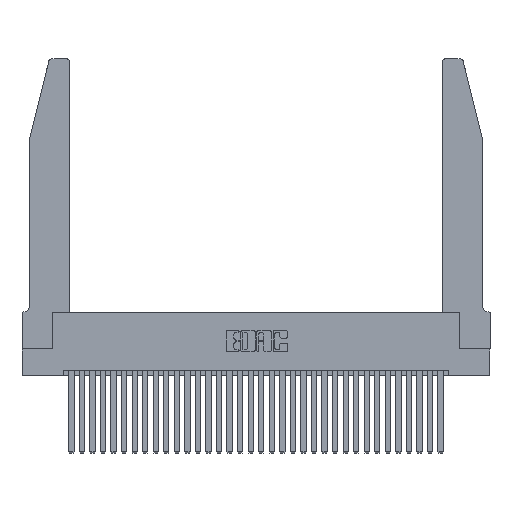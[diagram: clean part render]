
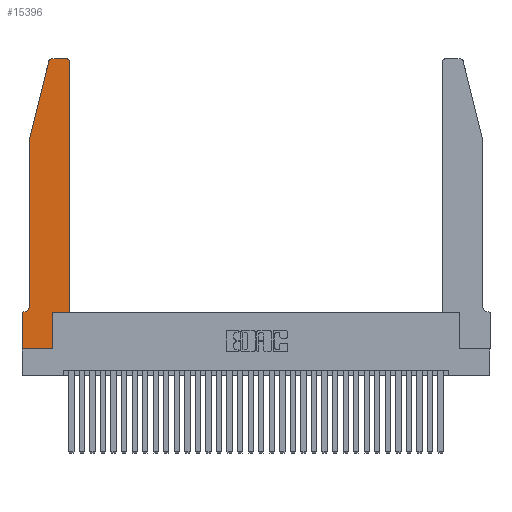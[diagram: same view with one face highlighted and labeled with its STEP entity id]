
A CAD part, top view. The second image highlights one B-rep face of the part: STEP entity #15396.
In plain terms, the highlighted planar face has unit normal (0, 0, 1).
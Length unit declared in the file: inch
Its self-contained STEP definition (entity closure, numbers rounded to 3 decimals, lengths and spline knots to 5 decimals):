
#211 = DIRECTION ( 'NONE',  ( 1., 0., 0. ) ) ;
#323 = DIRECTION ( 'NONE',  ( 1., 0., 0. ) ) ;
#579 = EDGE_CURVE ( 'NONE', #9746, #6793, #3070, .T. ) ;
#960 = ORIENTED_EDGE ( 'NONE', *, *, #579, .T. ) ;
#1198 = LINE ( 'NONE', #16739, #21111 ) ;
#2134 = DIRECTION ( 'NONE',  ( 0., 0., -1. ) ) ;
#2361 = EDGE_CURVE ( 'NONE', #6656, #9746, #30515, .T. ) ;
#2761 = EDGE_CURVE ( 'NONE', #21842, #29448, #1198, .T. ) ;
#3023 = CIRCLE ( 'NONE', #4635, 0.03 ) ;
#3070 = LINE ( 'NONE', #5357, #6378 ) ;
#3404 = CARTESIAN_POINT ( 'NONE',  ( 0., 0., 0.37 ) ) ;
#3480 = LINE ( 'NONE', #3404, #15290 ) ;
#3879 = DIRECTION ( 'NONE',  ( -1., 0., 0. ) ) ;
#4460 = DIRECTION ( 'NONE',  ( 0., 1., 0. ) ) ;
#4463 = CARTESIAN_POINT ( 'NONE',  ( 0., 0.35, 0.37 ) ) ;
#4635 = AXIS2_PLACEMENT_3D ( 'NONE', #15820, #31505, #323 ) ;
#4909 = DIRECTION ( 'NONE',  ( 1., 0., 0. ) ) ;
#5357 = CARTESIAN_POINT ( 'NONE',  ( 0.4505, 0.35, 0.37 ) ) ;
#6378 = VECTOR ( 'NONE', #23825, 39.37008 ) ;
#6656 = VERTEX_POINT ( 'NONE', #24664 ) ;
#6670 = CARTESIAN_POINT ( 'NONE',  ( 0.25487, 2.72718, 0.37 ) ) ;
#6793 = VERTEX_POINT ( 'NONE', #17738 ) ;
#7742 = CARTESIAN_POINT ( 'NONE',  ( 0.0055, 0.35, 0.37 ) ) ;
#8192 = DIRECTION ( 'NONE',  ( 0., 0., 1. ) ) ;
#8232 = ORIENTED_EDGE ( 'NONE', *, *, #32897, .T. ) ;
#9725 = CIRCLE ( 'NONE', #13963, 0.03 ) ;
#9746 = VERTEX_POINT ( 'NONE', #15189 ) ;
#9823 = VECTOR ( 'NONE', #10952, 39.37008 ) ;
#10944 = EDGE_CURVE ( 'NONE', #14311, #14879, #15466, .T. ) ;
#10952 = DIRECTION ( 'NONE',  ( -0.239, -0.971, 0. ) ) ;
#12093 = CARTESIAN_POINT ( 'NONE',  ( 0.4505, 0.35, 0.37 ) ) ;
#12300 = DIRECTION ( 'NONE',  ( 0., 0., 1. ) ) ;
#12455 = FACE_OUTER_BOUND ( 'NONE', #14557, .T. ) ;
#12748 = VERTEX_POINT ( 'NONE', #31370 ) ;
#13379 = ORIENTED_EDGE ( 'NONE', *, *, #23040, .T. ) ;
#13963 = AXIS2_PLACEMENT_3D ( 'NONE', #25676, #12300, #4909 ) ;
#14055 = CARTESIAN_POINT ( 'NONE',  ( 0.284, 2.75, 0.37 ) ) ;
#14167 = ORIENTED_EDGE ( 'NONE', *, *, #19040, .T. ) ;
#14311 = VERTEX_POINT ( 'NONE', #19934 ) ;
#14557 = EDGE_LOOP ( 'NONE', ( #19829, #8232, #14167, #31690, #17922, #22378, #33277, #13379, #32469, #960, #21387, #23759 ) ) ;
#14879 = VERTEX_POINT ( 'NONE', #31973 ) ;
#15189 = CARTESIAN_POINT ( 'NONE',  ( 0.2865, 0.35, 0.37 ) ) ;
#15290 = VECTOR ( 'NONE', #21895, 39.37008 ) ;
#15393 = VECTOR ( 'NONE', #4460, 39.37008 ) ;
#15396 = ADVANCED_FACE ( 'NONE', ( #12455 ), #27158, .T. ) ;
#15466 = LINE ( 'NONE', #17640, #18686 ) ;
#15694 = CARTESIAN_POINT ( 'NONE',  ( 0.2865, 0.35, 0.37 ) ) ;
#15798 = CARTESIAN_POINT ( 'NONE',  ( 0., 0., 0.37 ) ) ;
#15820 = CARTESIAN_POINT ( 'NONE',  ( 0.4205, 2.72, 0.37 ) ) ;
#15999 = DIRECTION ( 'NONE',  ( 1., 0., 0. ) ) ;
#16010 = LINE ( 'NONE', #15798, #17278 ) ;
#16063 = VERTEX_POINT ( 'NONE', #28778 ) ;
#16739 = CARTESIAN_POINT ( 'NONE',  ( 0.0755, 0.35, 0.37 ) ) ;
#17278 = VECTOR ( 'NONE', #211, 39.37008 ) ;
#17640 = CARTESIAN_POINT ( 'NONE',  ( 0.0755, 2., 0.37 ) ) ;
#17738 = CARTESIAN_POINT ( 'NONE',  ( 0.4505, 0.35, 0.37 ) ) ;
#17922 = ORIENTED_EDGE ( 'NONE', *, *, #31210, .T. ) ;
#18179 = DIRECTION ( 'NONE',  ( -1., 0., 0. ) ) ;
#18686 = VECTOR ( 'NONE', #30674, 39.37008 ) ;
#19040 = EDGE_CURVE ( 'NONE', #23728, #14311, #22784, .T. ) ;
#19522 = CIRCLE ( 'NONE', #24799, 0.07 ) ;
#19829 = ORIENTED_EDGE ( 'NONE', *, *, #20448, .T. ) ;
#19934 = CARTESIAN_POINT ( 'NONE',  ( 0.0755, 2., 0.37 ) ) ;
#20329 = DIRECTION ( 'NONE',  ( -1., 0., 0. ) ) ;
#20351 = EDGE_CURVE ( 'NONE', #6793, #16063, #26333, .T. ) ;
#20448 = EDGE_CURVE ( 'NONE', #12748, #31572, #27999, .T. ) ;
#20629 = VERTEX_POINT ( 'NONE', #30149 ) ;
#21042 = VECTOR ( 'NONE', #18179, 39.37008 ) ;
#21111 = VECTOR ( 'NONE', #3879, 39.37008 ) ;
#21227 = EDGE_CURVE ( 'NONE', #29448, #20629, #3480, .T. ) ;
#21387 = ORIENTED_EDGE ( 'NONE', *, *, #20351, .T. ) ;
#21842 = VERTEX_POINT ( 'NONE', #7742 ) ;
#21895 = DIRECTION ( 'NONE',  ( 0., -1., 0. ) ) ;
#21995 = EDGE_CURVE ( 'NONE', #16063, #12748, #3023, .T. ) ;
#22378 = ORIENTED_EDGE ( 'NONE', *, *, #2761, .T. ) ;
#22784 = LINE ( 'NONE', #30982, #9823 ) ;
#23040 = EDGE_CURVE ( 'NONE', #20629, #6656, #16010, .T. ) ;
#23728 = VERTEX_POINT ( 'NONE', #6670 ) ;
#23759 = ORIENTED_EDGE ( 'NONE', *, *, #21995, .T. ) ;
#23825 = DIRECTION ( 'NONE',  ( 1., 0., 0. ) ) ;
#24664 = CARTESIAN_POINT ( 'NONE',  ( 0.2865, 0., 0.37 ) ) ;
#24799 = AXIS2_PLACEMENT_3D ( 'NONE', #25563, #2134, #20329 ) ;
#25563 = CARTESIAN_POINT ( 'NONE',  ( 0.0055, 0.42, 0.37 ) ) ;
#25676 = CARTESIAN_POINT ( 'NONE',  ( 0.284, 2.72, 0.37 ) ) ;
#26333 = LINE ( 'NONE', #12093, #15393 ) ;
#27158 = PLANE ( 'NONE',  #28894 ) ;
#27669 = VECTOR ( 'NONE', #31583, 39.37008 ) ;
#27999 = LINE ( 'NONE', #30887, #21042 ) ;
#28778 = CARTESIAN_POINT ( 'NONE',  ( 0.4505, 2.72, 0.37 ) ) ;
#28894 = AXIS2_PLACEMENT_3D ( 'NONE', #4463, #8192, #15999 ) ;
#29448 = VERTEX_POINT ( 'NONE', #30834 ) ;
#30149 = CARTESIAN_POINT ( 'NONE',  ( 0., 0., 0.37 ) ) ;
#30515 = LINE ( 'NONE', #15694, #27669 ) ;
#30674 = DIRECTION ( 'NONE',  ( 0., -1., 0. ) ) ;
#30834 = CARTESIAN_POINT ( 'NONE',  ( 0., 0.35, 0.37 ) ) ;
#30887 = CARTESIAN_POINT ( 'NONE',  ( 0.2605, 2.75, 0.37 ) ) ;
#30982 = CARTESIAN_POINT ( 'NONE',  ( 0.0755, 2., 0.37 ) ) ;
#31210 = EDGE_CURVE ( 'NONE', #14879, #21842, #19522, .T. ) ;
#31370 = CARTESIAN_POINT ( 'NONE',  ( 0.4205, 2.75, 0.37 ) ) ;
#31505 = DIRECTION ( 'NONE',  ( 0., 0., 1. ) ) ;
#31572 = VERTEX_POINT ( 'NONE', #14055 ) ;
#31583 = DIRECTION ( 'NONE',  ( 0., 1., 0. ) ) ;
#31690 = ORIENTED_EDGE ( 'NONE', *, *, #10944, .T. ) ;
#31973 = CARTESIAN_POINT ( 'NONE',  ( 0.0755, 0.42, 0.37 ) ) ;
#32469 = ORIENTED_EDGE ( 'NONE', *, *, #2361, .T. ) ;
#32897 = EDGE_CURVE ( 'NONE', #31572, #23728, #9725, .T. ) ;
#33277 = ORIENTED_EDGE ( 'NONE', *, *, #21227, .T. ) ;
